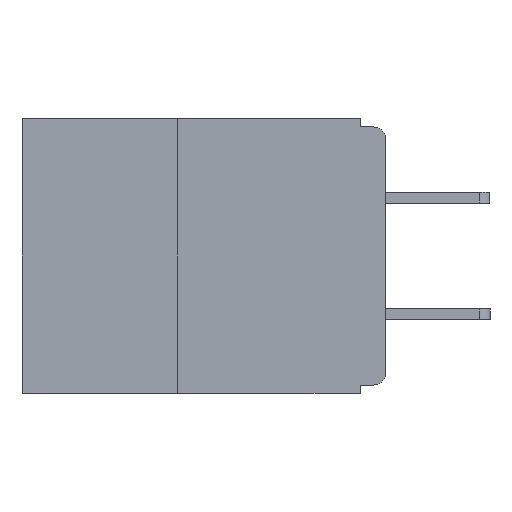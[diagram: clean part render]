
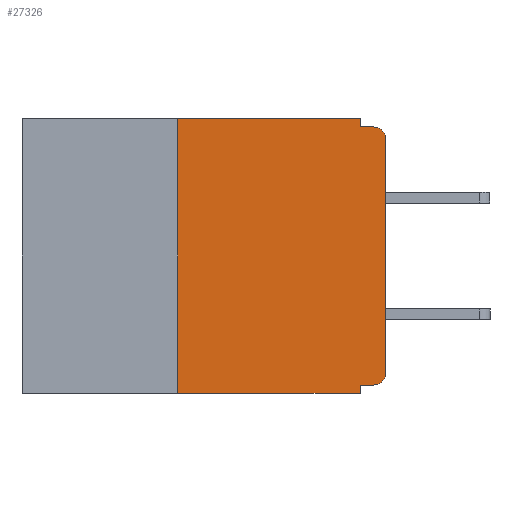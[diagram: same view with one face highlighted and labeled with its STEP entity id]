
A CAD part, left-side view. The second image highlights one B-rep face of the part: STEP entity #27326.
In plain terms, the highlighted planar face has unit normal (-1, 0, 0).
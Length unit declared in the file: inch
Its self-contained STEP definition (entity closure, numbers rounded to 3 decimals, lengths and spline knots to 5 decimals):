
#236 = ORIENTED_EDGE ( 'NONE', *, *, #2921, .T. ) ;
#274 = ORIENTED_EDGE ( 'NONE', *, *, #27270, .T. ) ;
#750 = CIRCLE ( 'NONE', #10981, 0.015 ) ;
#1253 = CARTESIAN_POINT ( 'NONE',  ( 0., 0.25, 0. ) ) ;
#1765 = VECTOR ( 'NONE', #14579, 39.37008 ) ;
#1821 = VECTOR ( 'NONE', #15280, 39.37008 ) ;
#2030 = CARTESIAN_POINT ( 'NONE',  ( 0., 0.015, -0.025 ) ) ;
#2921 = EDGE_CURVE ( 'NONE', #11203, #25828, #16662, .T. ) ;
#3488 = EDGE_CURVE ( 'NONE', #25828, #26443, #750, .T. ) ;
#3832 = DIRECTION ( 'NONE',  ( -1., 0., 0. ) ) ;
#4279 = DIRECTION ( 'NONE',  ( 0., 0., -1. ) ) ;
#4764 = VERTEX_POINT ( 'NONE', #15115 ) ;
#5088 = CARTESIAN_POINT ( 'NONE',  ( 0., 0.25, -0.33 ) ) ;
#5506 = LINE ( 'NONE', #19166, #17096 ) ;
#5791 = EDGE_CURVE ( 'NONE', #19184, #14112, #13093, .T. ) ;
#6147 = DIRECTION ( 'NONE',  ( 0., -1., 0. ) ) ;
#6334 = DIRECTION ( 'NONE',  ( 1., 0., 0. ) ) ;
#6371 = FACE_OUTER_BOUND ( 'NONE', #19633, .T. ) ;
#7313 = EDGE_CURVE ( 'NONE', #15084, #14112, #16688, .T. ) ;
#7314 = VECTOR ( 'NONE', #9897, 39.37008 ) ;
#7947 = VECTOR ( 'NONE', #19077, 39.37008 ) ;
#8097 = EDGE_CURVE ( 'NONE', #21598, #19184, #13653, .T. ) ;
#8306 = CARTESIAN_POINT ( 'NONE',  ( 0., 0.25, -0.33 ) ) ;
#9212 = DIRECTION ( 'NONE',  ( 0., -1., 0. ) ) ;
#9668 = VECTOR ( 'NONE', #9212, 39.37008 ) ;
#9897 = DIRECTION ( 'NONE',  ( 0., 0., -1. ) ) ;
#10826 = ORIENTED_EDGE ( 'NONE', *, *, #5791, .F. ) ;
#10904 = CARTESIAN_POINT ( 'NONE',  ( 0., 0.031, -0.33 ) ) ;
#10981 = AXIS2_PLACEMENT_3D ( 'NONE', #2030, #17424, #4279 ) ;
#11203 = VERTEX_POINT ( 'NONE', #16730 ) ;
#11791 = ORIENTED_EDGE ( 'NONE', *, *, #8097, .F. ) ;
#11821 = ORIENTED_EDGE ( 'NONE', *, *, #16010, .F. ) ;
#12546 = DIRECTION ( 'NONE',  ( 0., 0., 1. ) ) ;
#13093 = LINE ( 'NONE', #24784, #7314 ) ;
#13114 = CARTESIAN_POINT ( 'NONE',  ( 0., 0., -0.32 ) ) ;
#13653 = LINE ( 'NONE', #13114, #1821 ) ;
#13771 = DIRECTION ( 'NONE',  ( 0., 0., 1. ) ) ;
#14112 = VERTEX_POINT ( 'NONE', #10904 ) ;
#14281 = CIRCLE ( 'NONE', #14749, 0.015 ) ;
#14579 = DIRECTION ( 'NONE',  ( 0., 0., -1. ) ) ;
#14607 = EDGE_CURVE ( 'NONE', #15084, #25229, #27010, .T. ) ;
#14724 = VERTEX_POINT ( 'NONE', #23798 ) ;
#14749 = AXIS2_PLACEMENT_3D ( 'NONE', #16983, #3832, #19160 ) ;
#14776 = CARTESIAN_POINT ( 'NONE',  ( 0., 0.437, -0.33 ) ) ;
#14847 = ORIENTED_EDGE ( 'NONE', *, *, #3488, .T. ) ;
#15024 = PLANE ( 'NONE',  #24777 ) ;
#15084 = VERTEX_POINT ( 'NONE', #5088 ) ;
#15115 = CARTESIAN_POINT ( 'NONE',  ( 0., 0.031, -0.01 ) ) ;
#15187 = ORIENTED_EDGE ( 'NONE', *, *, #7313, .T. ) ;
#15193 = CARTESIAN_POINT ( 'NONE',  ( 0., 0.015, -0.32 ) ) ;
#15280 = DIRECTION ( 'NONE',  ( 0., 1., 0. ) ) ;
#15686 = VECTOR ( 'NONE', #12546, 39.37008 ) ;
#16002 = VECTOR ( 'NONE', #13771, 39.37008 ) ;
#16010 = EDGE_CURVE ( 'NONE', #14724, #4764, #24964, .T. ) ;
#16630 = CARTESIAN_POINT ( 'NONE',  ( 0., 0.031, -0.32 ) ) ;
#16662 = LINE ( 'NONE', #25059, #16002 ) ;
#16685 = CARTESIAN_POINT ( 'NONE',  ( 0., 0.031, 0. ) ) ;
#16688 = LINE ( 'NONE', #14776, #7947 ) ;
#16730 = CARTESIAN_POINT ( 'NONE',  ( 0., 0., -0.305 ) ) ;
#16983 = CARTESIAN_POINT ( 'NONE',  ( 0., 0.015, -0.305 ) ) ;
#17096 = VECTOR ( 'NONE', #6147, 39.37008 ) ;
#17424 = DIRECTION ( 'NONE',  ( -1., 0., 0. ) ) ;
#18199 = EDGE_CURVE ( 'NONE', #4764, #26443, #21055, .T. ) ;
#18875 = ORIENTED_EDGE ( 'NONE', *, *, #24689, .F. ) ;
#19077 = DIRECTION ( 'NONE',  ( 0., -1., 0. ) ) ;
#19160 = DIRECTION ( 'NONE',  ( 0., 0., -1. ) ) ;
#19166 = CARTESIAN_POINT ( 'NONE',  ( 0., 0.437, 0. ) ) ;
#19184 = VERTEX_POINT ( 'NONE', #16630 ) ;
#19330 = CARTESIAN_POINT ( 'NONE',  ( 0., 0.437, 0. ) ) ;
#19633 = EDGE_LOOP ( 'NONE', ( #236, #14847, #27495, #11821, #18875, #25876, #15187, #10826, #11791, #274 ) ) ;
#21055 = LINE ( 'NONE', #22052, #9668 ) ;
#21467 = DIRECTION ( 'NONE',  ( 0., 0., -1. ) ) ;
#21598 = VERTEX_POINT ( 'NONE', #15193 ) ;
#22052 = CARTESIAN_POINT ( 'NONE',  ( 0., 0., -0.01 ) ) ;
#23798 = CARTESIAN_POINT ( 'NONE',  ( 0., 0.031, 0. ) ) ;
#24689 = EDGE_CURVE ( 'NONE', #25229, #14724, #5506, .T. ) ;
#24777 = AXIS2_PLACEMENT_3D ( 'NONE', #19330, #6334, #21467 ) ;
#24784 = CARTESIAN_POINT ( 'NONE',  ( 0., 0.031, -0.33 ) ) ;
#24964 = LINE ( 'NONE', #16685, #1765 ) ;
#25024 = CARTESIAN_POINT ( 'NONE',  ( 0., 0.015, -0.01 ) ) ;
#25059 = CARTESIAN_POINT ( 'NONE',  ( 0., 0., 0. ) ) ;
#25229 = VERTEX_POINT ( 'NONE', #1253 ) ;
#25828 = VERTEX_POINT ( 'NONE', #27342 ) ;
#25876 = ORIENTED_EDGE ( 'NONE', *, *, #14607, .F. ) ;
#26443 = VERTEX_POINT ( 'NONE', #25024 ) ;
#27010 = LINE ( 'NONE', #8306, #15686 ) ;
#27270 = EDGE_CURVE ( 'NONE', #21598, #11203, #14281, .T. ) ;
#27326 = ADVANCED_FACE ( 'NONE', ( #6371 ), #15024, .F. ) ;
#27342 = CARTESIAN_POINT ( 'NONE',  ( 0., 0., -0.025 ) ) ;
#27495 = ORIENTED_EDGE ( 'NONE', *, *, #18199, .F. ) ;
